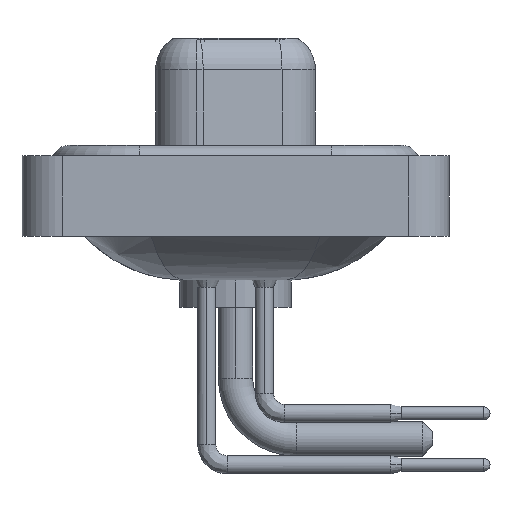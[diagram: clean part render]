
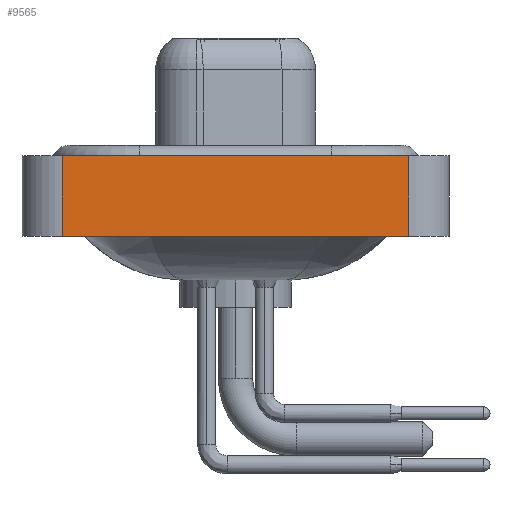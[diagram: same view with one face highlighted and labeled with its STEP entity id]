
A CAD part, left-side view. The second image highlights one B-rep face of the part: STEP entity #9565.
In plain terms, the highlighted planar face has unit normal (-1, 0, 0).
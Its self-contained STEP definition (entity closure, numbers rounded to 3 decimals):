
#1284 = VECTOR ( 'NONE', #11831, 1000. ) ;
#2845 = CARTESIAN_POINT ( 'NONE',  ( -7.3, -8.55, 0.4 ) ) ;
#3087 = ORIENTED_EDGE ( 'NONE', *, *, #22221, .T. ) ;
#3732 = DIRECTION ( 'NONE',  ( 0., -1., 0. ) ) ;
#4611 = DIRECTION ( 'NONE',  ( 0., 0., 1. ) ) ;
#5171 = EDGE_CURVE ( 'NONE', #20022, #19459, #6673, .T. ) ;
#5275 = VERTEX_POINT ( 'NONE', #21981 ) ;
#6673 = LINE ( 'NONE', #18821, #1284 ) ;
#7571 = CARTESIAN_POINT ( 'NONE',  ( -7.3, 8.55, -3.6 ) ) ;
#8145 = ORIENTED_EDGE ( 'NONE', *, *, #5171, .T. ) ;
#8223 = PLANE ( 'NONE',  #21764 ) ;
#9565 = ADVANCED_FACE ( 'NONE', ( #9906 ), #8223, .T. ) ;
#9880 = ORIENTED_EDGE ( 'NONE', *, *, #12338, .F. ) ;
#9906 = FACE_OUTER_BOUND ( 'NONE', #21440, .T. ) ;
#10570 = VECTOR ( 'NONE', #21992, 1000. ) ;
#10712 = CARTESIAN_POINT ( 'NONE',  ( -7.3, -8.55, -3.6 ) ) ;
#11202 = CARTESIAN_POINT ( 'NONE',  ( -7.3, 8.55, -3.6 ) ) ;
#11218 = CARTESIAN_POINT ( 'NONE',  ( -7.3, -8.55, -3.6 ) ) ;
#11831 = DIRECTION ( 'NONE',  ( 0., 0., 1. ) ) ;
#12338 = EDGE_CURVE ( 'NONE', #22096, #5275, #21666, .T. ) ;
#12808 = VECTOR ( 'NONE', #3732, 1000. ) ;
#13289 = CARTESIAN_POINT ( 'NONE',  ( -7.3, -8.55, -3.6 ) ) ;
#14823 = LINE ( 'NONE', #2845, #19056 ) ;
#17457 = ORIENTED_EDGE ( 'NONE', *, *, #21381, .F. ) ;
#17792 = LINE ( 'NONE', #10712, #12808 ) ;
#18345 = DIRECTION ( 'NONE',  ( -1., 0., 0. ) ) ;
#18409 = DIRECTION ( 'NONE',  ( 0., -1., 0. ) ) ;
#18821 = CARTESIAN_POINT ( 'NONE',  ( -7.3, -8.55, -3.6 ) ) ;
#19056 = VECTOR ( 'NONE', #18409, 1000. ) ;
#19459 = VERTEX_POINT ( 'NONE', #21901 ) ;
#20022 = VERTEX_POINT ( 'NONE', #11218 ) ;
#21381 = EDGE_CURVE ( 'NONE', #5275, #19459, #14823, .T. ) ;
#21440 = EDGE_LOOP ( 'NONE', ( #8145, #17457, #9880, #3087 ) ) ;
#21666 = LINE ( 'NONE', #11202, #10570 ) ;
#21764 = AXIS2_PLACEMENT_3D ( 'NONE', #13289, #18345, #4611 ) ;
#21901 = CARTESIAN_POINT ( 'NONE',  ( -7.3, -8.55, 0.4 ) ) ;
#21981 = CARTESIAN_POINT ( 'NONE',  ( -7.3, 8.55, 0.4 ) ) ;
#21992 = DIRECTION ( 'NONE',  ( 0., 0., 1. ) ) ;
#22096 = VERTEX_POINT ( 'NONE', #7571 ) ;
#22221 = EDGE_CURVE ( 'NONE', #22096, #20022, #17792, .T. ) ;
